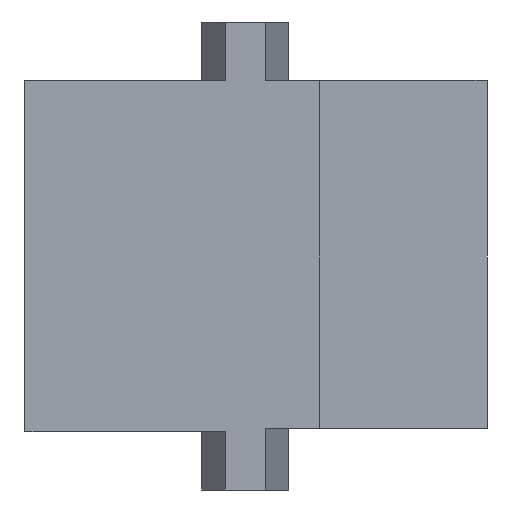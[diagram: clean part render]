
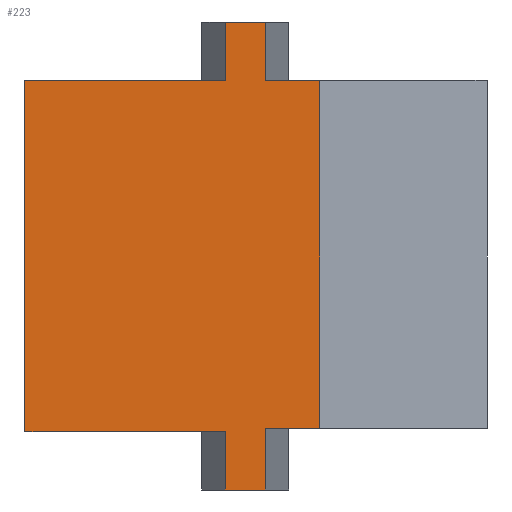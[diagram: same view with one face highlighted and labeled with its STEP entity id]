
A CAD part, left-side view. The second image highlights one B-rep face of the part: STEP entity #223.
In plain terms, the highlighted planar face has unit normal (-1, 0, 0).
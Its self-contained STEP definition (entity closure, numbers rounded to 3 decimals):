
#4 = EDGE_CURVE ( 'NONE', #226, #21, #15, .T. ) ;
#7 = CARTESIAN_POINT ( 'NONE',  ( -0.985, 8.204, 13.351 ) ) ;
#15 = LINE ( 'NONE', #277, #58 ) ;
#16 = CARTESIAN_POINT ( 'NONE',  ( -0.985, 3.442, 4.726 ) ) ;
#21 = VERTEX_POINT ( 'NONE', #478 ) ;
#29 = VECTOR ( 'NONE', #333, 1000. ) ;
#35 = EDGE_CURVE ( 'NONE', #528, #673, #271, .T. ) ;
#55 = CARTESIAN_POINT ( 'NONE',  ( -0.985, 0.265, 7.269 ) ) ;
#58 = VECTOR ( 'NONE', #798, 1000. ) ;
#65 = EDGE_CURVE ( 'NONE', #197, #226, #754, .T. ) ;
#68 = ORIENTED_EDGE ( 'NONE', *, *, #200, .T. ) ;
#75 = VECTOR ( 'NONE', #368, 1000. ) ;
#84 = DIRECTION ( 'NONE',  ( 0., -1., 0. ) ) ;
#85 = DIRECTION ( 'NONE',  ( 0., 0., 1. ) ) ;
#95 = VERTEX_POINT ( 'NONE', #569 ) ;
#110 = EDGE_CURVE ( 'NONE', #644, #197, #691, .T. ) ;
#124 = EDGE_CURVE ( 'NONE', #203, #823, #817, .T. ) ;
#131 = CARTESIAN_POINT ( 'NONE',  ( -0.985, 3.442, -6.299 ) ) ;
#143 = LINE ( 'NONE', #7, #452 ) ;
#156 = ORIENTED_EDGE ( 'NONE', *, *, #505, .F. ) ;
#173 = CARTESIAN_POINT ( 'NONE',  ( -0.985, 0.265, -4.643 ) ) ;
#197 = VERTEX_POINT ( 'NONE', #431 ) ;
#200 = EDGE_CURVE ( 'NONE', #379, #21, #683, .T. ) ;
#203 = VERTEX_POINT ( 'NONE', #426 ) ;
#210 = VECTOR ( 'NONE', #304, 1000. ) ;
#215 = DIRECTION ( 'NONE',  ( 0., -1., 0. ) ) ;
#223 = ADVANCED_FACE ( 'NONE', ( #564 ), #726, .F. ) ;
#226 = VERTEX_POINT ( 'NONE', #173 ) ;
#271 = LINE ( 'NONE', #716, #29 ) ;
#277 = CARTESIAN_POINT ( 'NONE',  ( -0.985, 1.102, -4.643 ) ) ;
#280 = CARTESIAN_POINT ( 'NONE',  ( -0.985, 1.732, 7.269 ) ) ;
#282 = CARTESIAN_POINT ( 'NONE',  ( -0.985, 10.804, 7.269 ) ) ;
#301 = DIRECTION ( 'NONE',  ( 1., 0., 0. ) ) ;
#304 = DIRECTION ( 'NONE',  ( 0., -1., 0. ) ) ;
#311 = ORIENTED_EDGE ( 'NONE', *, *, #773, .T. ) ;
#332 = CARTESIAN_POINT ( 'NONE',  ( -0.985, 2.812, -6.299 ) ) ;
#333 = DIRECTION ( 'NONE',  ( 0., 0., -1. ) ) ;
#334 = CARTESIAN_POINT ( 'NONE',  ( -0.985, 10.804, -4.724 ) ) ;
#354 = CARTESIAN_POINT ( 'NONE',  ( -0.985, 8.204, -4.724 ) ) ;
#356 = ORIENTED_EDGE ( 'NONE', *, *, #638, .F. ) ;
#368 = DIRECTION ( 'NONE',  ( 0., 0., -1. ) ) ;
#374 = VECTOR ( 'NONE', #85, 1000. ) ;
#379 = VERTEX_POINT ( 'NONE', #486 ) ;
#386 = DIRECTION ( 'NONE',  ( 0., 1., 0. ) ) ;
#395 = VECTOR ( 'NONE', #215, 1000. ) ;
#397 = VECTOR ( 'NONE', #386, 1000. ) ;
#403 = VECTOR ( 'NONE', #815, 1000. ) ;
#406 = LINE ( 'NONE', #833, #586 ) ;
#413 = LINE ( 'NONE', #16, #395 ) ;
#426 = CARTESIAN_POINT ( 'NONE',  ( -0.985, 2.812, -4.724 ) ) ;
#431 = CARTESIAN_POINT ( 'NONE',  ( -0.985, 0.265, 4.726 ) ) ;
#437 = CARTESIAN_POINT ( 'NONE',  ( -0.985, 2.812, 7.269 ) ) ;
#446 = AXIS2_PLACEMENT_3D ( 'NONE', #282, #301, #496 ) ;
#452 = VECTOR ( 'NONE', #791, 1000. ) ;
#455 = EDGE_CURVE ( 'NONE', #203, #766, #583, .T. ) ;
#458 = CARTESIAN_POINT ( 'NONE',  ( -0.985, 2.812, 6.301 ) ) ;
#478 = CARTESIAN_POINT ( 'NONE',  ( -0.985, 1.732, -4.643 ) ) ;
#479 = ORIENTED_EDGE ( 'NONE', *, *, #110, .F. ) ;
#481 = EDGE_CURVE ( 'NONE', #95, #673, #413, .T. ) ;
#486 = CARTESIAN_POINT ( 'NONE',  ( -0.985, 1.732, -6.299 ) ) ;
#493 = ORIENTED_EDGE ( 'NONE', *, *, #4, .F. ) ;
#496 = DIRECTION ( 'NONE',  ( 0., 1., 0. ) ) ;
#505 = EDGE_CURVE ( 'NONE', #528, #759, #406, .T. ) ;
#528 = VERTEX_POINT ( 'NONE', #458 ) ;
#564 = FACE_OUTER_BOUND ( 'NONE', #603, .T. ) ;
#569 = CARTESIAN_POINT ( 'NONE',  ( -0.985, 8.204, 4.726 ) ) ;
#583 = LINE ( 'NONE', #334, #397 ) ;
#586 = VECTOR ( 'NONE', #84, 1000. ) ;
#603 = EDGE_LOOP ( 'NONE', ( #710, #311, #826, #652, #356, #68, #493, #834, #479, #728, #156, #663 ) ) ;
#623 = CARTESIAN_POINT ( 'NONE',  ( -0.985, 1.732, 7.269 ) ) ;
#633 = VECTOR ( 'NONE', #646, 1000. ) ;
#638 = EDGE_CURVE ( 'NONE', #379, #823, #707, .T. ) ;
#644 = VERTEX_POINT ( 'NONE', #779 ) ;
#646 = DIRECTION ( 'NONE',  ( 0., 1., 0. ) ) ;
#652 = ORIENTED_EDGE ( 'NONE', *, *, #124, .T. ) ;
#663 = ORIENTED_EDGE ( 'NONE', *, *, #35, .T. ) ;
#673 = VERTEX_POINT ( 'NONE', #676 ) ;
#676 = CARTESIAN_POINT ( 'NONE',  ( -0.985, 2.812, 4.726 ) ) ;
#683 = LINE ( 'NONE', #623, #403 ) ;
#691 = LINE ( 'NONE', #820, #210 ) ;
#699 = EDGE_CURVE ( 'NONE', #644, #759, #736, .T. ) ;
#707 = LINE ( 'NONE', #131, #633 ) ;
#710 = ORIENTED_EDGE ( 'NONE', *, *, #481, .F. ) ;
#716 = CARTESIAN_POINT ( 'NONE',  ( -0.985, 2.812, 7.269 ) ) ;
#726 = PLANE ( 'NONE',  #446 ) ;
#728 = ORIENTED_EDGE ( 'NONE', *, *, #699, .T. ) ;
#736 = LINE ( 'NONE', #280, #374 ) ;
#750 = DIRECTION ( 'NONE',  ( 0., 0., -1. ) ) ;
#754 = LINE ( 'NONE', #55, #829 ) ;
#759 = VERTEX_POINT ( 'NONE', #781 ) ;
#766 = VERTEX_POINT ( 'NONE', #354 ) ;
#773 = EDGE_CURVE ( 'NONE', #95, #766, #143, .T. ) ;
#779 = CARTESIAN_POINT ( 'NONE',  ( -0.985, 1.732, 4.726 ) ) ;
#781 = CARTESIAN_POINT ( 'NONE',  ( -0.985, 1.732, 6.301 ) ) ;
#791 = DIRECTION ( 'NONE',  ( 0., 0., -1. ) ) ;
#798 = DIRECTION ( 'NONE',  ( 0., 1., 0. ) ) ;
#815 = DIRECTION ( 'NONE',  ( 0., 0., 1. ) ) ;
#817 = LINE ( 'NONE', #437, #75 ) ;
#820 = CARTESIAN_POINT ( 'NONE',  ( -0.985, 0.265, 4.726 ) ) ;
#823 = VERTEX_POINT ( 'NONE', #332 ) ;
#826 = ORIENTED_EDGE ( 'NONE', *, *, #455, .F. ) ;
#829 = VECTOR ( 'NONE', #750, 1000. ) ;
#833 = CARTESIAN_POINT ( 'NONE',  ( -0.985, 1.102, 6.301 ) ) ;
#834 = ORIENTED_EDGE ( 'NONE', *, *, #65, .F. ) ;
